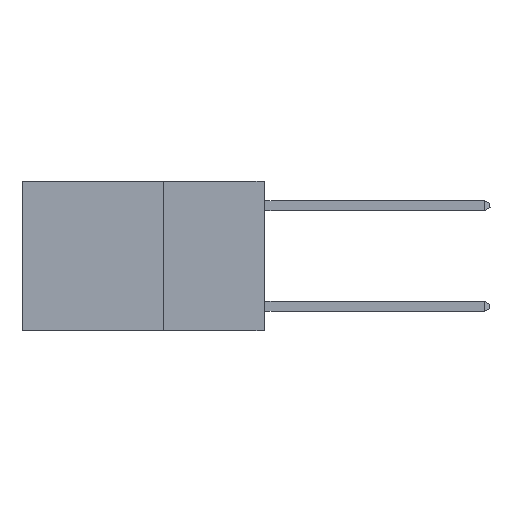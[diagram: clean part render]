
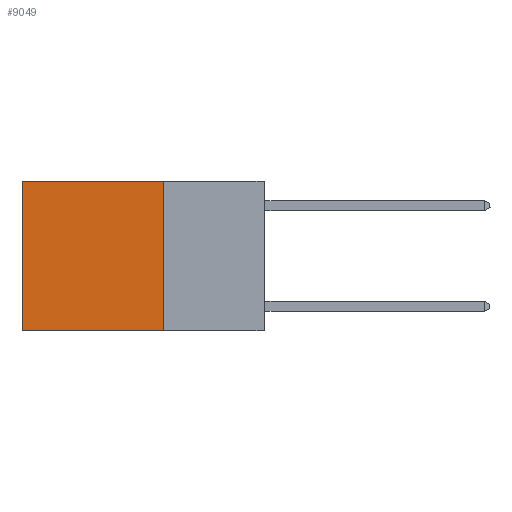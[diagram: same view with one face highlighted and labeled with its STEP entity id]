
A CAD part, left-side view. The second image highlights one B-rep face of the part: STEP entity #9049.
In plain terms, the highlighted planar face has unit normal (-1, 0, 0).
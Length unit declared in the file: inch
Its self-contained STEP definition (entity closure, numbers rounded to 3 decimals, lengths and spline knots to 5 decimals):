
#157 = CARTESIAN_POINT ( 'NONE',  ( 0.2625, 0.25, -0.37 ) ) ;
#371 = LINE ( 'NONE', #10695, #573 ) ;
#573 = VECTOR ( 'NONE', #8657, 39.37008 ) ;
#1009 = EDGE_CURVE ( 'NONE', #7905, #13172, #371, .T. ) ;
#2080 = EDGE_CURVE ( 'NONE', #3160, #11424, #12914, .T. ) ;
#2542 = CARTESIAN_POINT ( 'NONE',  ( 0.2625, 0.6, 0. ) ) ;
#2634 = DIRECTION ( 'NONE',  ( 0., 0., -1. ) ) ;
#2813 = PLANE ( 'NONE',  #13149 ) ;
#2920 = ORIENTED_EDGE ( 'NONE', *, *, #1009, .T. ) ;
#3160 = VERTEX_POINT ( 'NONE', #157 ) ;
#3193 = EDGE_LOOP ( 'NONE', ( #7662, #3543, #10734, #2920 ) ) ;
#3364 = CARTESIAN_POINT ( 'NONE',  ( 0.2625, 0.25, 0. ) ) ;
#3543 = ORIENTED_EDGE ( 'NONE', *, *, #2080, .F. ) ;
#3783 = DIRECTION ( 'NONE',  ( 0., 0., -1. ) ) ;
#4894 = DIRECTION ( 'NONE',  ( 0., 1., 0. ) ) ;
#5754 = EDGE_CURVE ( 'NONE', #13172, #11424, #9048, .T. ) ;
#5865 = CARTESIAN_POINT ( 'NONE',  ( 0.2625, 0.6, 0. ) ) ;
#5907 = FACE_OUTER_BOUND ( 'NONE', #3193, .T. ) ;
#5918 = CARTESIAN_POINT ( 'NONE',  ( 0.2625, 0.6, -0.37 ) ) ;
#6964 = CARTESIAN_POINT ( 'NONE',  ( 0.2625, 0.25, 0. ) ) ;
#7019 = VECTOR ( 'NONE', #2634, 39.37008 ) ;
#7112 = EDGE_CURVE ( 'NONE', #7905, #3160, #11892, .T. ) ;
#7662 = ORIENTED_EDGE ( 'NONE', *, *, #5754, .T. ) ;
#7905 = VERTEX_POINT ( 'NONE', #3364 ) ;
#8241 = VECTOR ( 'NONE', #4894, 39.37008 ) ;
#8657 = DIRECTION ( 'NONE',  ( 0., 1., 0. ) ) ;
#9048 = LINE ( 'NONE', #5865, #9443 ) ;
#9049 = ADVANCED_FACE ( 'NONE', ( #5907 ), #2813, .F. ) ;
#9443 = VECTOR ( 'NONE', #13136, 39.37008 ) ;
#10695 = CARTESIAN_POINT ( 'NONE',  ( 0.2625, 0.25, 0. ) ) ;
#10734 = ORIENTED_EDGE ( 'NONE', *, *, #7112, .F. ) ;
#11049 = DIRECTION ( 'NONE',  ( 1., 0., 0. ) ) ;
#11424 = VERTEX_POINT ( 'NONE', #5918 ) ;
#11892 = LINE ( 'NONE', #11965, #7019 ) ;
#11965 = CARTESIAN_POINT ( 'NONE',  ( 0.2625, 0.25, 0. ) ) ;
#12914 = LINE ( 'NONE', #13100, #8241 ) ;
#13100 = CARTESIAN_POINT ( 'NONE',  ( 0.2625, 0.25, -0.37 ) ) ;
#13136 = DIRECTION ( 'NONE',  ( 0., 0., -1. ) ) ;
#13149 = AXIS2_PLACEMENT_3D ( 'NONE', #6964, #11049, #3783 ) ;
#13172 = VERTEX_POINT ( 'NONE', #2542 ) ;
